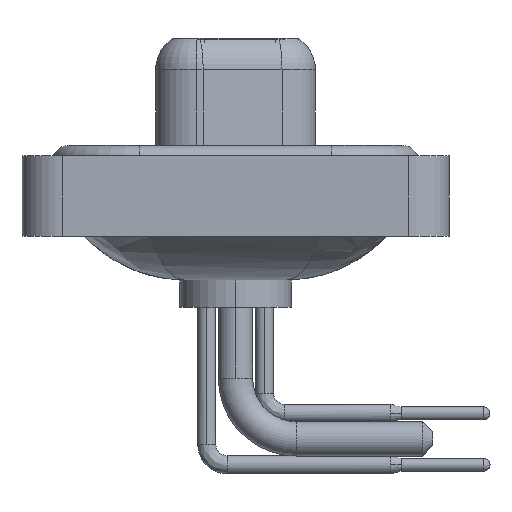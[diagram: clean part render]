
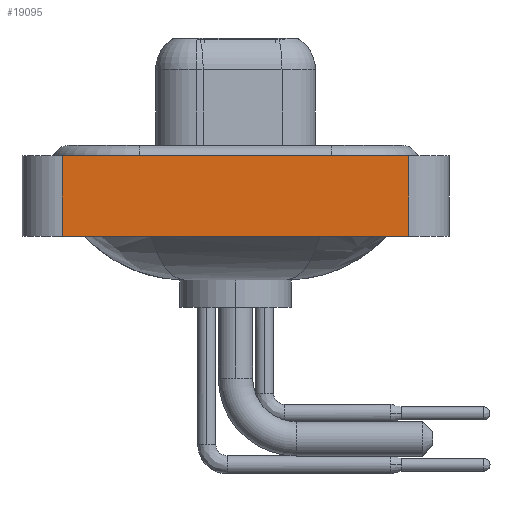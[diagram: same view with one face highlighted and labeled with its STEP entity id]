
A CAD part, left-side view. The second image highlights one B-rep face of the part: STEP entity #19095.
In plain terms, the highlighted planar face has unit normal (-1, 0, 0).
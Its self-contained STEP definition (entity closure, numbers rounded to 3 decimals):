
#1154 = CARTESIAN_POINT ( 'NONE',  ( -7.35, -8.55, -3.6 ) ) ;
#2019 = CARTESIAN_POINT ( 'NONE',  ( -7.35, -8.55, -3.6 ) ) ;
#2256 = EDGE_CURVE ( 'NONE', #11738, #18905, #6023, .T. ) ;
#2356 = PLANE ( 'NONE',  #9635 ) ;
#2692 = FACE_OUTER_BOUND ( 'NONE', #15803, .T. ) ;
#2933 = LINE ( 'NONE', #16945, #7066 ) ;
#3729 = ORIENTED_EDGE ( 'NONE', *, *, #20503, .F. ) ;
#3979 = VERTEX_POINT ( 'NONE', #19916 ) ;
#4162 = VERTEX_POINT ( 'NONE', #6598 ) ;
#4224 = VECTOR ( 'NONE', #8168, 1000. ) ;
#4488 = DIRECTION ( 'NONE',  ( 0., -1., 0. ) ) ;
#4622 = ORIENTED_EDGE ( 'NONE', *, *, #2256, .T. ) ;
#6023 = LINE ( 'NONE', #7866, #13029 ) ;
#6145 = DIRECTION ( 'NONE',  ( -1., 0., 0. ) ) ;
#6598 = CARTESIAN_POINT ( 'NONE',  ( -7.35, -8.55, 0.4 ) ) ;
#7066 = VECTOR ( 'NONE', #8249, 1000. ) ;
#7866 = CARTESIAN_POINT ( 'NONE',  ( -7.35, -8.55, -3.6 ) ) ;
#8168 = DIRECTION ( 'NONE',  ( 0., 0., 1. ) ) ;
#8249 = DIRECTION ( 'NONE',  ( 0., 0., 1. ) ) ;
#9035 = VECTOR ( 'NONE', #4488, 1000. ) ;
#9635 = AXIS2_PLACEMENT_3D ( 'NONE', #16373, #6145, #19930 ) ;
#9904 = LINE ( 'NONE', #18483, #9035 ) ;
#9969 = EDGE_CURVE ( 'NONE', #3979, #4162, #9904, .T. ) ;
#10903 = ORIENTED_EDGE ( 'NONE', *, *, #18399, .T. ) ;
#11738 = VERTEX_POINT ( 'NONE', #15473 ) ;
#13029 = VECTOR ( 'NONE', #21534, 1000. ) ;
#15322 = ORIENTED_EDGE ( 'NONE', *, *, #9969, .F. ) ;
#15473 = CARTESIAN_POINT ( 'NONE',  ( -7.35, 8.55, -3.6 ) ) ;
#15803 = EDGE_LOOP ( 'NONE', ( #10903, #15322, #3729, #4622 ) ) ;
#16373 = CARTESIAN_POINT ( 'NONE',  ( -7.35, -8.55, -3.6 ) ) ;
#16880 = LINE ( 'NONE', #1154, #4224 ) ;
#16945 = CARTESIAN_POINT ( 'NONE',  ( -7.35, 8.55, -3.6 ) ) ;
#18399 = EDGE_CURVE ( 'NONE', #18905, #4162, #16880, .T. ) ;
#18483 = CARTESIAN_POINT ( 'NONE',  ( -7.35, -8.55, 0.4 ) ) ;
#18905 = VERTEX_POINT ( 'NONE', #2019 ) ;
#19095 = ADVANCED_FACE ( 'NONE', ( #2692 ), #2356, .T. ) ;
#19916 = CARTESIAN_POINT ( 'NONE',  ( -7.35, 8.55, 0.4 ) ) ;
#19930 = DIRECTION ( 'NONE',  ( 0., 0., 1. ) ) ;
#20503 = EDGE_CURVE ( 'NONE', #11738, #3979, #2933, .T. ) ;
#21534 = DIRECTION ( 'NONE',  ( 0., -1., 0. ) ) ;
